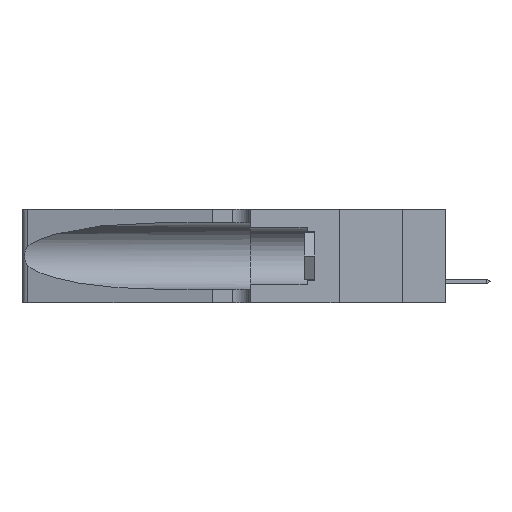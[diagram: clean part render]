
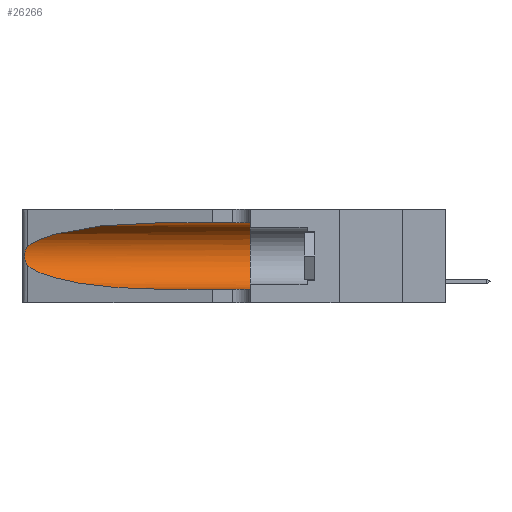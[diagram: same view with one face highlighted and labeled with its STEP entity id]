
A CAD part, left-side view. The second image highlights one B-rep face of the part: STEP entity #26266.
In plain terms, the highlighted cylindrical face has radius 3.308 mm (diameter 6.617 mm), a partial arc.
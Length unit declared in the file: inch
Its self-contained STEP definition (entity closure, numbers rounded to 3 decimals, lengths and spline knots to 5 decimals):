
#474 = DIRECTION ( 'NONE',  ( 0., -1., 0. ) ) ;
#1845 = CARTESIAN_POINT ( 'NONE',  ( 0.1305, 1.61858, 0.31525 ) ) ;
#1882 = VERTEX_POINT ( 'NONE', #23361 ) ;
#2466 = CARTESIAN_POINT ( 'NONE',  ( 0.1305, 0.35, 0.31525 ) ) ;
#2581 = LINE ( 'NONE', #1845, #8008 ) ;
#2936 = CARTESIAN_POINT ( 'NONE',  ( 0.1305, 0.72297, 0.31525 ) ) ;
#4692 = CARTESIAN_POINT ( 'NONE',  ( 0.25487, 1.22718, 0.14631 ) ) ;
#5398 = VERTEX_POINT ( 'NONE', #2466 ) ;
#5566 = CARTESIAN_POINT ( 'NONE',  ( 0.25639, 1.23186, 0.15144 ) ) ;
#6092 = CARTESIAN_POINT ( 'NONE',  ( 0.25487, 1.22718, 0.22369 ) ) ;
#6276 = CARTESIAN_POINT ( 'NONE',  ( 0.25487, 1.22718, 0.14631 ) ) ;
#6761 = CARTESIAN_POINT ( 'NONE',  ( 0.25487, 1.22718, 0.22369 ) ) ;
#6855 = VERTEX_POINT ( 'NONE', #12144 ) ;
#7992 =( BOUNDED_CURVE ( )  B_SPLINE_CURVE ( 3, ( #14042, #16078, #28349, #14247 ),
 .UNSPECIFIED., .F., .F. ) 
 B_SPLINE_CURVE_WITH_KNOTS ( ( 4, 4 ),
 ( 3.44316, 4.71239 ),
 .UNSPECIFIED. ) 
 CURVE ( )  GEOMETRIC_REPRESENTATION_ITEM ( )  RATIONAL_B_SPLINE_CURVE ( ( 1., 0.87, 0.87, 1. ) ) 
 REPRESENTATION_ITEM ( '' )  );
#8008 = VECTOR ( 'NONE', #15790, 39.37008 ) ;
#8578 = CARTESIAN_POINT ( 'NONE',  ( 0.26075, 1.23896, 0.19203 ) ) ;
#9019 = CARTESIAN_POINT ( 'NONE',  ( 0.26018, 1.23835, 0.19895 ) ) ;
#9279 = VERTEX_POINT ( 'NONE', #2936 ) ;
#9563 = CARTESIAN_POINT ( 'NONE',  ( 0.25789, 1.23486, 0.15765 ) ) ;
#9644 = DIRECTION ( 'NONE',  ( 0., 0., -1. ) ) ;
#10899 = DIRECTION ( 'NONE',  ( 0., 1., 0. ) ) ;
#12144 = CARTESIAN_POINT ( 'NONE',  ( 0.1305, 0.72297, 0.05475 ) ) ;
#12642 = VECTOR ( 'NONE', #474, 39.37008 ) ;
#12777 = CARTESIAN_POINT ( 'NONE',  ( 0.25555, 1.22993, 0.14849 ) ) ;
#12984 = CARTESIAN_POINT ( 'NONE',  ( 0.25639, 1.23184, 0.21858 ) ) ;
#13490 = CARTESIAN_POINT ( 'NONE',  ( 0.25854, 1.2359, 0.20912 ) ) ;
#13555 = FACE_OUTER_BOUND ( 'NONE', #26522, .T. ) ;
#14042 = CARTESIAN_POINT ( 'NONE',  ( 0.25487, 1.22718, 0.14631 ) ) ;
#14247 = CARTESIAN_POINT ( 'NONE',  ( 0.1305, 0.72297, 0.05475 ) ) ;
#15163 = LINE ( 'NONE', #16806, #12642 ) ;
#15518 = CARTESIAN_POINT ( 'NONE',  ( 0.25555, 1.22994, 0.2215 ) ) ;
#15790 = DIRECTION ( 'NONE',  ( 0., -1., 0. ) ) ;
#16037 = EDGE_CURVE ( 'NONE', #6855, #27989, #15163, .T. ) ;
#16078 = CARTESIAN_POINT ( 'NONE',  ( 0.2373, 1.15595, 0.08982 ) ) ;
#16144 = CIRCLE ( 'NONE', #23082, 0.13025 ) ;
#16806 = CARTESIAN_POINT ( 'NONE',  ( 0.1305, 1.61858, 0.05475 ) ) ;
#17083 = EDGE_CURVE ( 'NONE', #5398, #27989, #16144, .T. ) ;
#18558 = B_SPLINE_CURVE_WITH_KNOTS ( 'NONE', 3,
 ( #6092, #15518, #12984, #21964, #13490, #9019, #8578, #29201, #24676, #25158, #9563, #5566, #12777, #6276 ),
 .UNSPECIFIED., .F., .F.,
 ( 4, 2, 2, 2, 2, 2, 4 ),
 ( 0., 0.00027, 0.00053, 0.00107, 0.0016, 0.00187, 0.00214 ),
 .UNSPECIFIED. ) ;
#18802 = ORIENTED_EDGE ( 'NONE', *, *, #27519, .T. ) ;
#18942 =( BOUNDED_CURVE ( )  B_SPLINE_CURVE ( 3, ( #21487, #28439, #19308, #6761 ),
 .UNSPECIFIED., .F., .F. ) 
 B_SPLINE_CURVE_WITH_KNOTS ( ( 4, 4 ),
 ( 1.5708, 2.84003 ),
 .UNSPECIFIED. ) 
 CURVE ( )  GEOMETRIC_REPRESENTATION_ITEM ( )  RATIONAL_B_SPLINE_CURVE ( ( 1., 0.87, 0.87, 1. ) ) 
 REPRESENTATION_ITEM ( '' )  );
#19308 = CARTESIAN_POINT ( 'NONE',  ( 0.2373, 1.15595, 0.28018 ) ) ;
#20188 = CARTESIAN_POINT ( 'NONE',  ( 0.1305, 0.35, 0.05475 ) ) ;
#21487 = CARTESIAN_POINT ( 'NONE',  ( 0.1305, 0.72297, 0.31525 ) ) ;
#21902 = AXIS2_PLACEMENT_3D ( 'NONE', #24815, #26431, #9644 ) ;
#21964 = CARTESIAN_POINT ( 'NONE',  ( 0.25787, 1.23484, 0.2124 ) ) ;
#22099 = CYLINDRICAL_SURFACE ( 'NONE', #21902, 0.13025 ) ;
#22318 = CARTESIAN_POINT ( 'NONE',  ( 0.1305, 0.35, 0.185 ) ) ;
#22372 = EDGE_CURVE ( 'NONE', #1882, #26815, #18558, .T. ) ;
#22462 = ORIENTED_EDGE ( 'NONE', *, *, #28951, .T. ) ;
#22863 = ORIENTED_EDGE ( 'NONE', *, *, #22372, .T. ) ;
#23082 = AXIS2_PLACEMENT_3D ( 'NONE', #22318, #10899, #26959 ) ;
#23361 = CARTESIAN_POINT ( 'NONE',  ( 0.25487, 1.22718, 0.22369 ) ) ;
#23462 = EDGE_CURVE ( 'NONE', #9279, #5398, #2581, .T. ) ;
#24676 = CARTESIAN_POINT ( 'NONE',  ( 0.26017, 1.23833, 0.17102 ) ) ;
#24815 = CARTESIAN_POINT ( 'NONE',  ( 0.1305, 1.61858, 0.185 ) ) ;
#24999 = ORIENTED_EDGE ( 'NONE', *, *, #23462, .F. ) ;
#25158 = CARTESIAN_POINT ( 'NONE',  ( 0.25856, 1.23593, 0.16098 ) ) ;
#26266 = ADVANCED_FACE ( 'NONE', ( #13555 ), #22099, .F. ) ;
#26431 = DIRECTION ( 'NONE',  ( 0., -1., 0. ) ) ;
#26522 = EDGE_LOOP ( 'NONE', ( #22462, #22863, #18802, #29485, #29315, #24999 ) ) ;
#26815 = VERTEX_POINT ( 'NONE', #4692 ) ;
#26959 = DIRECTION ( 'NONE',  ( 0., 0., 1. ) ) ;
#27519 = EDGE_CURVE ( 'NONE', #26815, #6855, #7992, .T. ) ;
#27989 = VERTEX_POINT ( 'NONE', #20188 ) ;
#28349 = CARTESIAN_POINT ( 'NONE',  ( 0.18966, 0.96281, 0.05475 ) ) ;
#28439 = CARTESIAN_POINT ( 'NONE',  ( 0.18966, 0.96281, 0.31525 ) ) ;
#28951 = EDGE_CURVE ( 'NONE', #9279, #1882, #18942, .T. ) ;
#29201 = CARTESIAN_POINT ( 'NONE',  ( 0.26075, 1.23896, 0.178 ) ) ;
#29315 = ORIENTED_EDGE ( 'NONE', *, *, #17083, .F. ) ;
#29485 = ORIENTED_EDGE ( 'NONE', *, *, #16037, .T. ) ;
